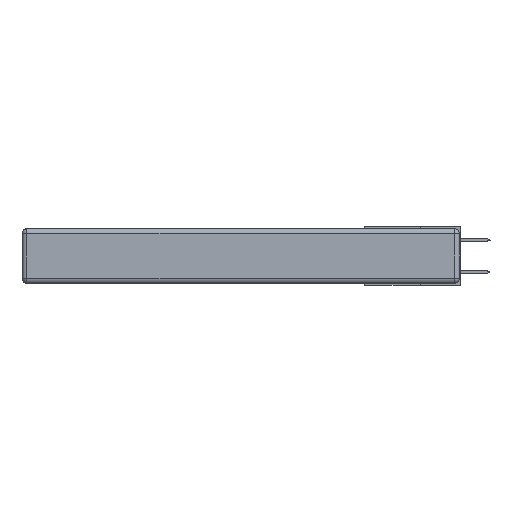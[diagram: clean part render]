
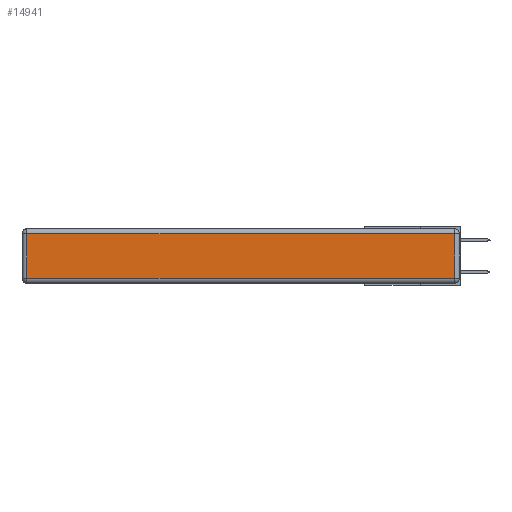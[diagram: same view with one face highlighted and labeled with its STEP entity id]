
A CAD part, left-side view. The second image highlights one B-rep face of the part: STEP entity #14941.
In plain terms, the highlighted planar face has unit normal (-1, 0, 0).
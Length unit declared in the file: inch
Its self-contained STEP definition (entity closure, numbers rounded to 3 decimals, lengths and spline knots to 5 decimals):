
#915 = CARTESIAN_POINT ( 'NONE',  ( 0., 0., -0.343 ) ) ;
#2501 = LINE ( 'NONE', #20667, #6609 ) ;
#2618 = VECTOR ( 'NONE', #9083, 39.37008 ) ;
#2681 = EDGE_CURVE ( 'NONE', #10773, #10847, #8241, .T. ) ;
#2746 = PLANE ( 'NONE',  #12587 ) ;
#3764 = ORIENTED_EDGE ( 'NONE', *, *, #16628, .T. ) ;
#5730 = VECTOR ( 'NONE', #18591, 39.37008 ) ;
#5792 = CARTESIAN_POINT ( 'NONE',  ( 0., 0.03, -0.03 ) ) ;
#5862 = CARTESIAN_POINT ( 'NONE',  ( 0., 0.03, -0.343 ) ) ;
#6609 = VECTOR ( 'NONE', #13920, 39.37008 ) ;
#7375 = VERTEX_POINT ( 'NONE', #11537 ) ;
#8047 = DIRECTION ( 'NONE',  ( -1., 0., 0. ) ) ;
#8241 = LINE ( 'NONE', #5862, #9840 ) ;
#8427 = CARTESIAN_POINT ( 'NONE',  ( 0., 2.72, -0.03 ) ) ;
#9083 = DIRECTION ( 'NONE',  ( 0., 1., 0. ) ) ;
#9452 = VERTEX_POINT ( 'NONE', #8427 ) ;
#9524 = DIRECTION ( 'NONE',  ( 0., 0., 1. ) ) ;
#9840 = VECTOR ( 'NONE', #9524, 39.37008 ) ;
#10773 = VERTEX_POINT ( 'NONE', #12886 ) ;
#10847 = VERTEX_POINT ( 'NONE', #5792 ) ;
#11537 = CARTESIAN_POINT ( 'NONE',  ( 0., 2.72, -0.313 ) ) ;
#12587 = AXIS2_PLACEMENT_3D ( 'NONE', #915, #8047, #19014 ) ;
#12886 = CARTESIAN_POINT ( 'NONE',  ( 0., 0.03, -0.313 ) ) ;
#13639 = LINE ( 'NONE', #20426, #5730 ) ;
#13711 = ORIENTED_EDGE ( 'NONE', *, *, #18755, .T. ) ;
#13920 = DIRECTION ( 'NONE',  ( 0., -1., 0. ) ) ;
#14242 = CARTESIAN_POINT ( 'NONE',  ( 0., 2.75, -0.03 ) ) ;
#14534 = ORIENTED_EDGE ( 'NONE', *, *, #2681, .T. ) ;
#14941 = ADVANCED_FACE ( 'NONE', ( #17678 ), #2746, .T. ) ;
#16628 = EDGE_CURVE ( 'NONE', #10847, #9452, #20293, .T. ) ;
#17678 = FACE_OUTER_BOUND ( 'NONE', #21350, .T. ) ;
#18591 = DIRECTION ( 'NONE',  ( 0., 0., -1. ) ) ;
#18755 = EDGE_CURVE ( 'NONE', #7375, #10773, #2501, .T. ) ;
#19014 = DIRECTION ( 'NONE',  ( 0., 0., 1. ) ) ;
#19525 = EDGE_CURVE ( 'NONE', #9452, #7375, #13639, .T. ) ;
#20138 = ORIENTED_EDGE ( 'NONE', *, *, #19525, .T. ) ;
#20293 = LINE ( 'NONE', #14242, #2618 ) ;
#20426 = CARTESIAN_POINT ( 'NONE',  ( 0., 2.72, -0.343 ) ) ;
#20667 = CARTESIAN_POINT ( 'NONE',  ( 0., 0., -0.313 ) ) ;
#21350 = EDGE_LOOP ( 'NONE', ( #13711, #14534, #3764, #20138 ) ) ;
